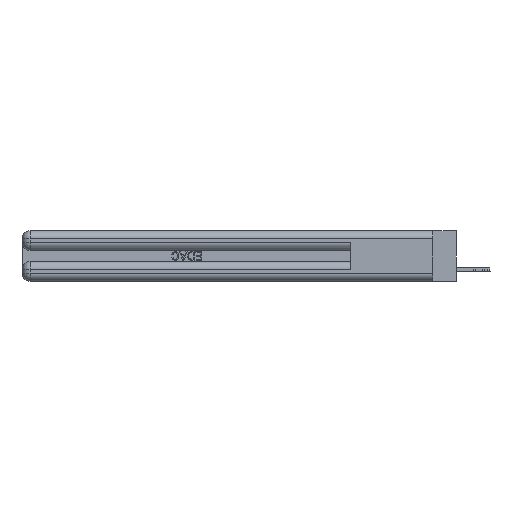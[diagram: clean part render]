
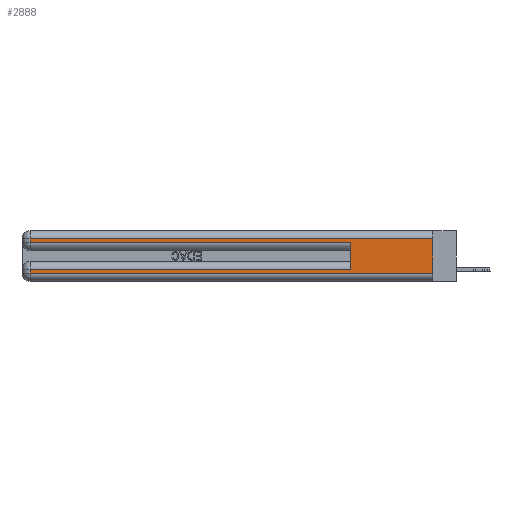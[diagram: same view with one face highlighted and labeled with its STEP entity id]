
A CAD part, left-side view. The second image highlights one B-rep face of the part: STEP entity #2888.
In plain terms, the highlighted planar face has unit normal (-1, 0, 0).
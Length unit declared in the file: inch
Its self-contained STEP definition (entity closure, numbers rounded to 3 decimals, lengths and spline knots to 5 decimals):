
#659 = ORIENTED_EDGE ( 'NONE', *, *, #27065, .T. ) ;
#1827 = FACE_OUTER_BOUND ( 'NONE', #16021, .T. ) ;
#2888 = ADVANCED_FACE ( 'NONE', ( #1827 ), #34301, .F. ) ;
#3591 = CARTESIAN_POINT ( 'NONE',  ( 0., 2.94, 0.285 ) ) ;
#4190 = DIRECTION ( 'NONE',  ( 0., 1., 0. ) ) ;
#9248 = VECTOR ( 'NONE', #38789, 39.37008 ) ;
#10560 = LINE ( 'NONE', #50494, #9248 ) ;
#10994 = CARTESIAN_POINT ( 'NONE',  ( 0., 2.94, 0.31 ) ) ;
#11103 = ORIENTED_EDGE ( 'NONE', *, *, #33446, .T. ) ;
#11756 = CARTESIAN_POINT ( 'NONE',  ( 0., 0., 0.06 ) ) ;
#12682 = CARTESIAN_POINT ( 'NONE',  ( 0., 0., 0.37 ) ) ;
#13077 = AXIS2_PLACEMENT_3D ( 'NONE', #12682, #29552, #17423 ) ;
#13626 = VECTOR ( 'NONE', #29015, 39.37008 ) ;
#14918 = DIRECTION ( 'NONE',  ( 0., 0., -1. ) ) ;
#15342 = VERTEX_POINT ( 'NONE', #46347 ) ;
#15861 = CARTESIAN_POINT ( 'NONE',  ( 0., 2.94, 0.085 ) ) ;
#16021 = EDGE_LOOP ( 'NONE', ( #44352, #40191, #45831, #659, #43994, #25514, #11103, #18347 ) ) ;
#17305 = LINE ( 'NONE', #34891, #48991 ) ;
#17423 = DIRECTION ( 'NONE',  ( 0., 0., -1. ) ) ;
#18010 = CARTESIAN_POINT ( 'NONE',  ( 0., 2.94, 0.37 ) ) ;
#18347 = ORIENTED_EDGE ( 'NONE', *, *, #32872, .T. ) ;
#18674 = CARTESIAN_POINT ( 'NONE',  ( 0., 0., 0.37 ) ) ;
#19174 = VERTEX_POINT ( 'NONE', #11756 ) ;
#19562 = DIRECTION ( 'NONE',  ( 0., -1., 0. ) ) ;
#20613 = VECTOR ( 'NONE', #39290, 39.37008 ) ;
#21208 = LINE ( 'NONE', #18010, #20613 ) ;
#23118 = EDGE_CURVE ( 'NONE', #48776, #28804, #29687, .T. ) ;
#23435 = CARTESIAN_POINT ( 'NONE',  ( 0., 2.94, 0.37 ) ) ;
#24358 = CARTESIAN_POINT ( 'NONE',  ( 0., 2.94, 0.06 ) ) ;
#24923 = VERTEX_POINT ( 'NONE', #29095 ) ;
#25514 = ORIENTED_EDGE ( 'NONE', *, *, #27193, .T. ) ;
#26733 = EDGE_CURVE ( 'NONE', #24923, #15342, #10560, .T. ) ;
#26919 = DIRECTION ( 'NONE',  ( 0., -1., 0. ) ) ;
#27065 = EDGE_CURVE ( 'NONE', #31864, #15342, #31815, .T. ) ;
#27193 = EDGE_CURVE ( 'NONE', #24923, #47079, #32526, .T. ) ;
#28804 = VERTEX_POINT ( 'NONE', #10994 ) ;
#29015 = DIRECTION ( 'NONE',  ( 0., 1., 0. ) ) ;
#29095 = CARTESIAN_POINT ( 'NONE',  ( 0., 0.6, 0.085 ) ) ;
#29552 = DIRECTION ( 'NONE',  ( 1., 0., 0. ) ) ;
#29687 = LINE ( 'NONE', #45026, #13626 ) ;
#29899 = CARTESIAN_POINT ( 'NONE',  ( 0., 0., 0.31 ) ) ;
#31815 = LINE ( 'NONE', #39858, #35678 ) ;
#31864 = VERTEX_POINT ( 'NONE', #3591 ) ;
#32526 = LINE ( 'NONE', #45310, #44262 ) ;
#32872 = EDGE_CURVE ( 'NONE', #33148, #19174, #17305, .T. ) ;
#33148 = VERTEX_POINT ( 'NONE', #24358 ) ;
#33446 = EDGE_CURVE ( 'NONE', #47079, #33148, #53635, .T. ) ;
#34301 = PLANE ( 'NONE',  #13077 ) ;
#34891 = CARTESIAN_POINT ( 'NONE',  ( 0., 0., 0.06 ) ) ;
#35678 = VECTOR ( 'NONE', #19562, 39.37008 ) ;
#37297 = EDGE_CURVE ( 'NONE', #48776, #19174, #37647, .T. ) ;
#37647 = LINE ( 'NONE', #18674, #54739 ) ;
#38789 = DIRECTION ( 'NONE',  ( 0., 0., 1. ) ) ;
#39290 = DIRECTION ( 'NONE',  ( 0., 0., -1. ) ) ;
#39858 = CARTESIAN_POINT ( 'NONE',  ( 0., 0., 0.285 ) ) ;
#40191 = ORIENTED_EDGE ( 'NONE', *, *, #23118, .T. ) ;
#43994 = ORIENTED_EDGE ( 'NONE', *, *, #26733, .F. ) ;
#44262 = VECTOR ( 'NONE', #4190, 39.37008 ) ;
#44352 = ORIENTED_EDGE ( 'NONE', *, *, #37297, .F. ) ;
#44625 = EDGE_CURVE ( 'NONE', #28804, #31864, #21208, .T. ) ;
#45026 = CARTESIAN_POINT ( 'NONE',  ( 0., 0., 0.31 ) ) ;
#45310 = CARTESIAN_POINT ( 'NONE',  ( 0., 0., 0.085 ) ) ;
#45831 = ORIENTED_EDGE ( 'NONE', *, *, #44625, .T. ) ;
#46347 = CARTESIAN_POINT ( 'NONE',  ( 0., 0.6, 0.285 ) ) ;
#46965 = VECTOR ( 'NONE', #14918, 39.37008 ) ;
#47079 = VERTEX_POINT ( 'NONE', #15861 ) ;
#48230 = DIRECTION ( 'NONE',  ( 0., 0., -1. ) ) ;
#48776 = VERTEX_POINT ( 'NONE', #29899 ) ;
#48991 = VECTOR ( 'NONE', #26919, 39.37008 ) ;
#50494 = CARTESIAN_POINT ( 'NONE',  ( 0., 0.6, 0.145 ) ) ;
#53635 = LINE ( 'NONE', #23435, #46965 ) ;
#54739 = VECTOR ( 'NONE', #48230, 39.37008 ) ;
